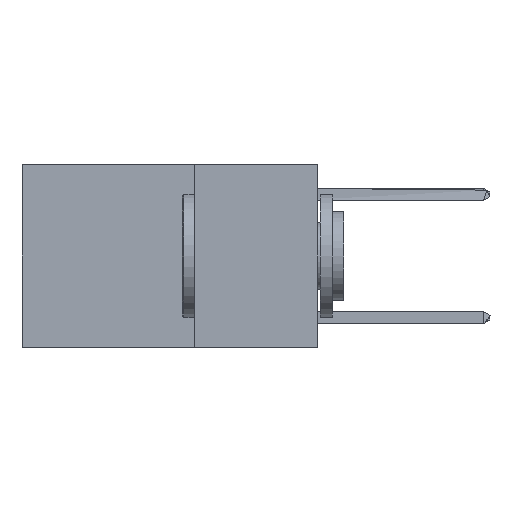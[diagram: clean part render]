
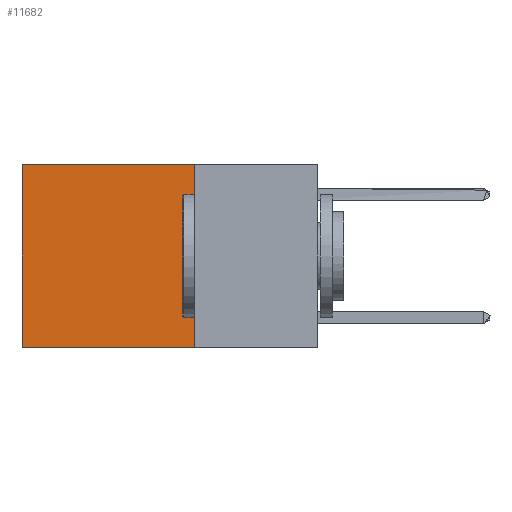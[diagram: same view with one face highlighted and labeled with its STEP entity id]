
A CAD part, left-side view. The second image highlights one B-rep face of the part: STEP entity #11682.
In plain terms, the highlighted planar face has unit normal (-1, 0, 0).
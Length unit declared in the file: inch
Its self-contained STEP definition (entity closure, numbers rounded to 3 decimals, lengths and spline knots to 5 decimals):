
#41 = ORIENTED_EDGE ( 'NONE', *, *, #13679, .T. ) ;
#157 = LINE ( 'NONE', #15342, #758 ) ;
#647 = DIRECTION ( 'NONE',  ( 0., 1., 0. ) ) ;
#758 = VECTOR ( 'NONE', #18950, 39.37008 ) ;
#1076 = LINE ( 'NONE', #13459, #15106 ) ;
#3521 = VERTEX_POINT ( 'NONE', #5914 ) ;
#3643 = EDGE_CURVE ( 'NONE', #7122, #22017, #1076, .T. ) ;
#4400 = EDGE_CURVE ( 'NONE', #7122, #7148, #157, .T. ) ;
#4950 = ORIENTED_EDGE ( 'NONE', *, *, #19099, .F. ) ;
#5102 = DIRECTION ( 'NONE',  ( 0., 0., -1. ) ) ;
#5141 = LINE ( 'NONE', #14158, #18515 ) ;
#5914 = CARTESIAN_POINT ( 'NONE',  ( 0.2625, 0.6, -0.37 ) ) ;
#6015 = ORIENTED_EDGE ( 'NONE', *, *, #3643, .T. ) ;
#7122 = VERTEX_POINT ( 'NONE', #9032 ) ;
#7148 = VERTEX_POINT ( 'NONE', #21598 ) ;
#8431 = LINE ( 'NONE', #15759, #12093 ) ;
#8976 = ORIENTED_EDGE ( 'NONE', *, *, #4400, .F. ) ;
#9032 = CARTESIAN_POINT ( 'NONE',  ( 0.2625, 0.25, 0. ) ) ;
#9343 = PLANE ( 'NONE',  #14377 ) ;
#10312 = DIRECTION ( 'NONE',  ( 0., 1., 0. ) ) ;
#11128 = DIRECTION ( 'NONE',  ( 0., 0., -1. ) ) ;
#11682 = ADVANCED_FACE ( 'NONE', ( #15802 ), #9343, .F. ) ;
#12093 = VECTOR ( 'NONE', #10312, 39.37008 ) ;
#13459 = CARTESIAN_POINT ( 'NONE',  ( 0.2625, 0.25, 0. ) ) ;
#13679 = EDGE_CURVE ( 'NONE', #22017, #3521, #5141, .T. ) ;
#13878 = CARTESIAN_POINT ( 'NONE',  ( 0.2625, 0.6, 0. ) ) ;
#14158 = CARTESIAN_POINT ( 'NONE',  ( 0.2625, 0.6, 0. ) ) ;
#14377 = AXIS2_PLACEMENT_3D ( 'NONE', #18341, #21803, #11128 ) ;
#15106 = VECTOR ( 'NONE', #647, 39.37008 ) ;
#15342 = CARTESIAN_POINT ( 'NONE',  ( 0.2625, 0.25, 0. ) ) ;
#15759 = CARTESIAN_POINT ( 'NONE',  ( 0.2625, 0.25, -0.37 ) ) ;
#15802 = FACE_OUTER_BOUND ( 'NONE', #20247, .T. ) ;
#18341 = CARTESIAN_POINT ( 'NONE',  ( 0.2625, 0.25, 0. ) ) ;
#18515 = VECTOR ( 'NONE', #5102, 39.37008 ) ;
#18950 = DIRECTION ( 'NONE',  ( 0., 0., -1. ) ) ;
#19099 = EDGE_CURVE ( 'NONE', #7148, #3521, #8431, .T. ) ;
#20247 = EDGE_LOOP ( 'NONE', ( #41, #4950, #8976, #6015 ) ) ;
#21598 = CARTESIAN_POINT ( 'NONE',  ( 0.2625, 0.25, -0.37 ) ) ;
#21803 = DIRECTION ( 'NONE',  ( 1., 0., 0. ) ) ;
#22017 = VERTEX_POINT ( 'NONE', #13878 ) ;
